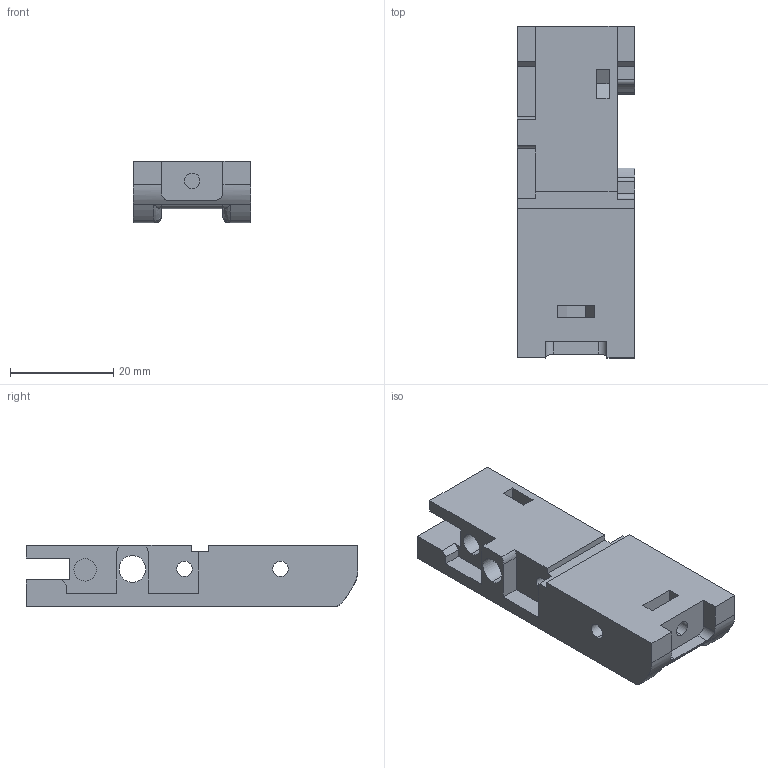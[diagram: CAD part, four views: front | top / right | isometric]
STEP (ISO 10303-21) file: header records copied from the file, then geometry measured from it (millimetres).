
FILE_DESCRIPTION (( 'STEP AP214' ), '1' );
FILE_NAME ('Thunderbolt_Mag_Well_Rear.STEP', '2021-09-12T03:40:00', ( '' ), ( '' ), 'SwSTEP 2.0', 'SolidWorks 2020', '' );
FILE_SCHEMA (( 'AUTOMOTIVE_DESIGN' ));
Length unit declared in the file: millimetre
Products named in the file (1): Thunderbolt_Mag_Well_Rear
Bounding box: 22.81 x 64.36 x 11.93 mm (x, y, z)
Volume: 10401.9 mm3; surface area: 6622.9 mm2
Topology: 1 solids, 1 shells, 103 faces, 287 edges, 187 vertices
Faces by surface type: plane 58, cylinder 33, bspline 12
Entity records: 3504 total; most frequent: CARTESIAN_POINT 856, ORIENTED_EDGE 570, DIRECTION 503, EDGE_CURVE 285, LINE 197, VECTOR 197, VERTEX_POINT 187, AXIS2_PLACEMENT_3D 153
